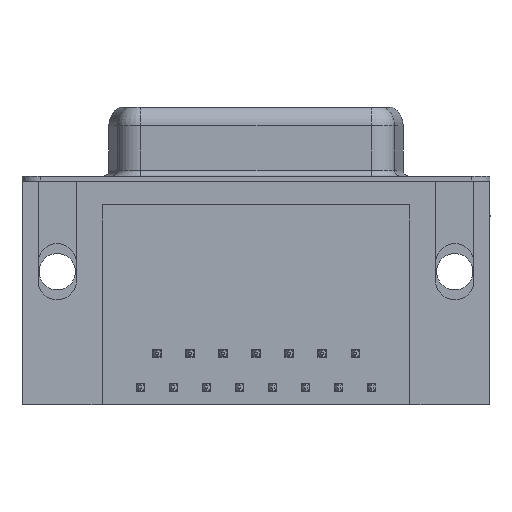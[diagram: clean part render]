
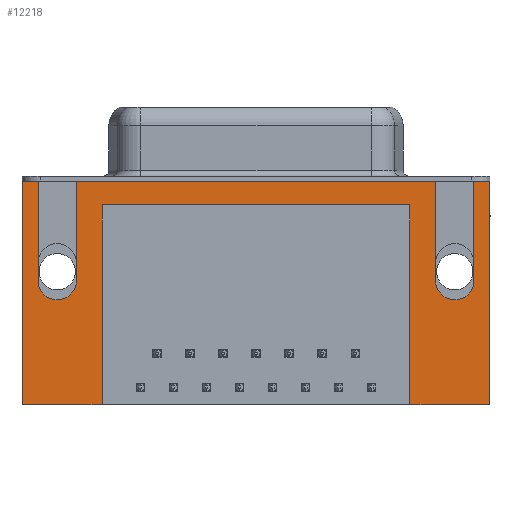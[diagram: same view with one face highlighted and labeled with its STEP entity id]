
A CAD part, front view. The second image highlights one B-rep face of the part: STEP entity #12218.
In plain terms, the highlighted planar face has unit normal (0, -1, 0).
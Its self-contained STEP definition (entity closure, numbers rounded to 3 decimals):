
#555 = PLANE ( 'NONE',  #1388 ) ;
#603 = CARTESIAN_POINT ( 'NONE',  ( -1.6, -6.275, -8.35 ) ) ;
#818 = VERTEX_POINT ( 'NONE', #22385 ) ;
#834 = EDGE_CURVE ( 'NONE', #23652, #12247, #22395, .T. ) ;
#953 = EDGE_CURVE ( 'NONE', #12247, #14101, #21598, .T. ) ;
#1106 = FACE_OUTER_BOUND ( 'NONE', #11823, .T. ) ;
#1326 = DIRECTION ( 'NONE',  ( 0., 0., 1. ) ) ;
#1369 = ORIENTED_EDGE ( 'NONE', *, *, #5999, .F. ) ;
#1372 = CARTESIAN_POINT ( 'NONE',  ( 31.72, -6.275, 0. ) ) ;
#1388 = AXIS2_PLACEMENT_3D ( 'NONE', #23188, #14704, #2579 ) ;
#1878 = CARTESIAN_POINT ( 'NONE',  ( 1.6, -6.275, 0. ) ) ;
#1956 = VERTEX_POINT ( 'NONE', #1372 ) ;
#2147 = ORIENTED_EDGE ( 'NONE', *, *, #13574, .F. ) ;
#2158 = DIRECTION ( 'NONE',  ( 0., 0., -1. ) ) ;
#2163 = VERTEX_POINT ( 'NONE', #603 ) ;
#2295 = ORIENTED_EDGE ( 'NONE', *, *, #834, .F. ) ;
#2511 = CARTESIAN_POINT ( 'NONE',  ( 36.255, -6.275, -2.5 ) ) ;
#2579 = DIRECTION ( 'NONE',  ( 0., 0., -1. ) ) ;
#3579 = CARTESIAN_POINT ( 'NONE',  ( 31.72, -6.275, 0. ) ) ;
#4125 = DIRECTION ( 'NONE',  ( -1., 0., 0. ) ) ;
#4240 = VERTEX_POINT ( 'NONE', #21119 ) ;
#4270 = ORIENTED_EDGE ( 'NONE', *, *, #8474, .F. ) ;
#4284 = VERTEX_POINT ( 'NONE', #25262 ) ;
#4670 = EDGE_CURVE ( 'NONE', #4284, #25802, #9402, .T. ) ;
#5110 = LINE ( 'NONE', #2511, #5160 ) ;
#5160 = VECTOR ( 'NONE', #1326, 1000. ) ;
#5522 = LINE ( 'NONE', #8573, #5610 ) ;
#5551 = CARTESIAN_POINT ( 'NONE',  ( -2.935, -6.275, 0. ) ) ;
#5610 = VECTOR ( 'NONE', #6483, 1000. ) ;
#5719 = VERTEX_POINT ( 'NONE', #26423 ) ;
#5947 = ORIENTED_EDGE ( 'NONE', *, *, #953, .F. ) ;
#5999 = EDGE_CURVE ( 'NONE', #25802, #5719, #5522, .T. ) ;
#6092 = EDGE_CURVE ( 'NONE', #19578, #18898, #5110, .T. ) ;
#6140 = CARTESIAN_POINT ( 'NONE',  ( 31.72, -6.275, -8.35 ) ) ;
#6451 = ORIENTED_EDGE ( 'NONE', *, *, #10015, .F. ) ;
#6483 = DIRECTION ( 'NONE',  ( 1., 0., 0. ) ) ;
#6500 = ORIENTED_EDGE ( 'NONE', *, *, #8824, .F. ) ;
#6676 = CARTESIAN_POINT ( 'NONE',  ( 36.255, -6.275, -18.76 ) ) ;
#6763 = DIRECTION ( 'NONE',  ( 0., -1., 0. ) ) ;
#6830 = CARTESIAN_POINT ( 'NONE',  ( 3.765, -6.275, -2. ) ) ;
#7517 = DIRECTION ( 'NONE',  ( 0., 0., -1. ) ) ;
#7620 = EDGE_CURVE ( 'NONE', #818, #10449, #24937, .T. ) ;
#7627 = ORIENTED_EDGE ( 'NONE', *, *, #9157, .F. ) ;
#7667 = VERTEX_POINT ( 'NONE', #23696 ) ;
#7820 = EDGE_CURVE ( 'NONE', #1956, #23652, #23785, .T. ) ;
#7835 = CARTESIAN_POINT ( 'NONE',  ( 3.765, -6.275, -18.76 ) ) ;
#7899 = VECTOR ( 'NONE', #25368, 1000. ) ;
#7999 = ORIENTED_EDGE ( 'NONE', *, *, #7820, .F. ) ;
#8003 = LINE ( 'NONE', #19223, #7899 ) ;
#8086 = CARTESIAN_POINT ( 'NONE',  ( 36.255, -6.275, -18.76 ) ) ;
#8146 = EDGE_CURVE ( 'NONE', #13627, #4284, #22246, .T. ) ;
#8474 = EDGE_CURVE ( 'NONE', #5719, #2163, #20181, .T. ) ;
#8573 = CARTESIAN_POINT ( 'NONE',  ( -2.935, -6.275, 0. ) ) ;
#8824 = EDGE_CURVE ( 'NONE', #24207, #13627, #18183, .T. ) ;
#8993 = CARTESIAN_POINT ( 'NONE',  ( 0., -6.275, -8.35 ) ) ;
#9157 = EDGE_CURVE ( 'NONE', #4240, #24207, #16027, .T. ) ;
#9232 = VECTOR ( 'NONE', #9857, 1000. ) ;
#9354 = EDGE_CURVE ( 'NONE', #7667, #4240, #14726, .T. ) ;
#9402 = LINE ( 'NONE', #9888, #9232 ) ;
#9658 = CARTESIAN_POINT ( 'NONE',  ( 36.255, -6.275, -18.76 ) ) ;
#9857 = DIRECTION ( 'NONE',  ( 0., 0., 1. ) ) ;
#9888 = CARTESIAN_POINT ( 'NONE',  ( -2.935, -6.275, -2.5 ) ) ;
#10015 = EDGE_CURVE ( 'NONE', #19578, #7667, #11643, .T. ) ;
#10230 = CARTESIAN_POINT ( 'NONE',  ( 36.255, -6.275, 0. ) ) ;
#10449 = VERTEX_POINT ( 'NONE', #1878 ) ;
#10794 = DIRECTION ( 'NONE',  ( 0., 0., 1. ) ) ;
#10816 = AXIS2_PLACEMENT_3D ( 'NONE', #8993, #23828, #11068 ) ;
#11068 = DIRECTION ( 'NONE',  ( 1., 0., 0. ) ) ;
#11643 = LINE ( 'NONE', #8086, #11688 ) ;
#11688 = VECTOR ( 'NONE', #4125, 1000. ) ;
#11823 = EDGE_LOOP ( 'NONE', ( #5947, #2295, #7999, #17433, #26170, #15438, #4270, #1369, #12052, #16718, #6500, #7627, #24019, #6451, #16009, #2147 ) ) ;
#11847 = DIRECTION ( 'NONE',  ( 0., 0., 1. ) ) ;
#12052 = ORIENTED_EDGE ( 'NONE', *, *, #4670, .F. ) ;
#12061 = CARTESIAN_POINT ( 'NONE',  ( -1.6, -6.275, 0. ) ) ;
#12149 = CARTESIAN_POINT ( 'NONE',  ( 34.92, -6.275, 0. ) ) ;
#12218 = ADVANCED_FACE ( 'NONE', ( #1106 ), #555, .T. ) ;
#12247 = VERTEX_POINT ( 'NONE', #14911 ) ;
#13355 = CARTESIAN_POINT ( 'NONE',  ( 3.765, -6.275, -2. ) ) ;
#13574 = EDGE_CURVE ( 'NONE', #14101, #18898, #19197, .T. ) ;
#13627 = VERTEX_POINT ( 'NONE', #7835 ) ;
#13827 = CARTESIAN_POINT ( 'NONE',  ( -2.935, -6.275, 0. ) ) ;
#13937 = EDGE_CURVE ( 'NONE', #2163, #818, #18116, .T. ) ;
#14101 = VERTEX_POINT ( 'NONE', #22261 ) ;
#14704 = DIRECTION ( 'NONE',  ( 0., -1., 0. ) ) ;
#14726 = LINE ( 'NONE', #23575, #14748 ) ;
#14748 = VECTOR ( 'NONE', #10794, 1000. ) ;
#14911 = CARTESIAN_POINT ( 'NONE',  ( 34.92, -6.275, -8.35 ) ) ;
#15175 = CARTESIAN_POINT ( 'NONE',  ( 1.6, -6.275, 0. ) ) ;
#15438 = ORIENTED_EDGE ( 'NONE', *, *, #13937, .F. ) ;
#15566 = DIRECTION ( 'NONE',  ( -1., 0., 0. ) ) ;
#15795 = VECTOR ( 'NONE', #15566, 1000. ) ;
#16009 = ORIENTED_EDGE ( 'NONE', *, *, #6092, .T. ) ;
#16027 = LINE ( 'NONE', #13355, #15795 ) ;
#16718 = ORIENTED_EDGE ( 'NONE', *, *, #8146, .F. ) ;
#16897 = EDGE_CURVE ( 'NONE', #10449, #1956, #8003, .T. ) ;
#17185 = DIRECTION ( 'NONE',  ( -1., 0., 0. ) ) ;
#17412 = DIRECTION ( 'NONE',  ( 0., 0., 1. ) ) ;
#17433 = ORIENTED_EDGE ( 'NONE', *, *, #16897, .F. ) ;
#18116 = CIRCLE ( 'NONE', #10816, 1.6 ) ;
#18183 = LINE ( 'NONE', #22330, #18738 ) ;
#18738 = VECTOR ( 'NONE', #7517, 1000. ) ;
#18898 = VERTEX_POINT ( 'NONE', #10230 ) ;
#19146 = VECTOR ( 'NONE', #22388, 1000. ) ;
#19197 = LINE ( 'NONE', #5551, #19146 ) ;
#19223 = CARTESIAN_POINT ( 'NONE',  ( -2.935, -6.275, 0. ) ) ;
#19578 = VERTEX_POINT ( 'NONE', #9658 ) ;
#20116 = VECTOR ( 'NONE', #2158, 1000. ) ;
#20181 = LINE ( 'NONE', #12061, #20116 ) ;
#20268 = DIRECTION ( 'NONE',  ( 0., 0., -1. ) ) ;
#21119 = CARTESIAN_POINT ( 'NONE',  ( 29.555, -6.275, -2. ) ) ;
#21551 = VECTOR ( 'NONE', #11847, 1000. ) ;
#21598 = LINE ( 'NONE', #12149, #21551 ) ;
#22087 = VECTOR ( 'NONE', #17185, 1000. ) ;
#22246 = LINE ( 'NONE', #6676, #22087 ) ;
#22261 = CARTESIAN_POINT ( 'NONE',  ( 34.92, -6.275, 0. ) ) ;
#22330 = CARTESIAN_POINT ( 'NONE',  ( 3.765, -6.275, -2. ) ) ;
#22385 = CARTESIAN_POINT ( 'NONE',  ( 1.6, -6.275, -8.35 ) ) ;
#22388 = DIRECTION ( 'NONE',  ( 1., 0., 0. ) ) ;
#22395 = CIRCLE ( 'NONE', #24054, 1.6 ) ;
#22833 = DIRECTION ( 'NONE',  ( -1., 0., 0. ) ) ;
#23188 = CARTESIAN_POINT ( 'NONE',  ( -2.935, -6.275, -2.5 ) ) ;
#23285 = CARTESIAN_POINT ( 'NONE',  ( 33.32, -6.275, -8.35 ) ) ;
#23575 = CARTESIAN_POINT ( 'NONE',  ( 29.555, -6.275, -2. ) ) ;
#23652 = VERTEX_POINT ( 'NONE', #6140 ) ;
#23696 = CARTESIAN_POINT ( 'NONE',  ( 29.555, -6.275, -18.76 ) ) ;
#23761 = VECTOR ( 'NONE', #20268, 1000. ) ;
#23785 = LINE ( 'NONE', #3579, #23761 ) ;
#23828 = DIRECTION ( 'NONE',  ( 0., -1., 0. ) ) ;
#24019 = ORIENTED_EDGE ( 'NONE', *, *, #9354, .F. ) ;
#24054 = AXIS2_PLACEMENT_3D ( 'NONE', #23285, #6763, #22833 ) ;
#24207 = VERTEX_POINT ( 'NONE', #6830 ) ;
#24816 = VECTOR ( 'NONE', #17412, 1000. ) ;
#24937 = LINE ( 'NONE', #15175, #24816 ) ;
#25262 = CARTESIAN_POINT ( 'NONE',  ( -2.935, -6.275, -18.76 ) ) ;
#25368 = DIRECTION ( 'NONE',  ( 1., 0., 0. ) ) ;
#25802 = VERTEX_POINT ( 'NONE', #13827 ) ;
#26170 = ORIENTED_EDGE ( 'NONE', *, *, #7620, .F. ) ;
#26423 = CARTESIAN_POINT ( 'NONE',  ( -1.6, -6.275, 0. ) ) ;
